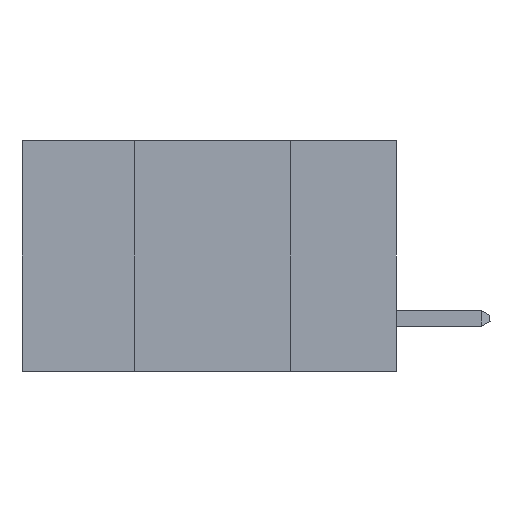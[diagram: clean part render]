
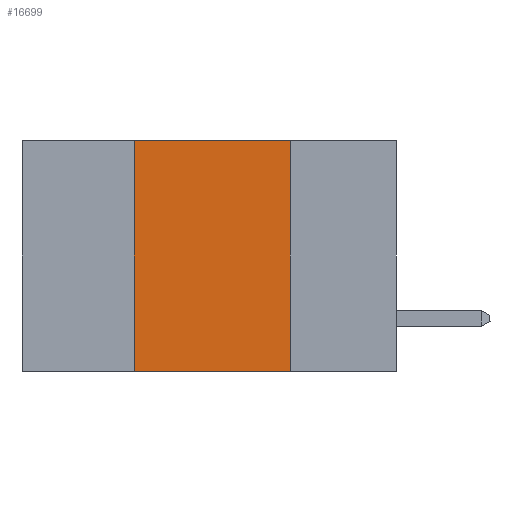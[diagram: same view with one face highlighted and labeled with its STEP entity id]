
A CAD part, left-side view. The second image highlights one B-rep face of the part: STEP entity #16699.
In plain terms, the highlighted planar face has unit normal (-1, 0, 0).
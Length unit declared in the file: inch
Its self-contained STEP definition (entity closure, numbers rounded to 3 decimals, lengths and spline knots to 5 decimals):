
#1188 = VECTOR ( 'NONE', #10572, 39.37008 ) ;
#1836 = ORIENTED_EDGE ( 'NONE', *, *, #16787, .T. ) ;
#1976 = CARTESIAN_POINT ( 'NONE',  ( 0., 0.6, 0. ) ) ;
#2512 = CARTESIAN_POINT ( 'NONE',  ( 0., 0.17, 0. ) ) ;
#2566 = LINE ( 'NONE', #2838, #17258 ) ;
#2645 = DIRECTION ( 'NONE',  ( 1., 0., 0. ) ) ;
#2838 = CARTESIAN_POINT ( 'NONE',  ( 0., 0.6, -0.37 ) ) ;
#2973 = CARTESIAN_POINT ( 'NONE',  ( 0., 0.17, 0. ) ) ;
#5061 = DIRECTION ( 'NONE',  ( 0., 0., 1. ) ) ;
#5926 = EDGE_CURVE ( 'NONE', #7946, #16697, #14800, .T. ) ;
#6313 = LINE ( 'NONE', #2973, #1188 ) ;
#7632 = ORIENTED_EDGE ( 'NONE', *, *, #9331, .F. ) ;
#7685 = DIRECTION ( 'NONE',  ( 0., -1., 0. ) ) ;
#7946 = VERTEX_POINT ( 'NONE', #13555 ) ;
#8011 = ORIENTED_EDGE ( 'NONE', *, *, #18366, .F. ) ;
#8271 = VECTOR ( 'NONE', #7685, 39.37008 ) ;
#9162 = CARTESIAN_POINT ( 'NONE',  ( 0., 0.17, -0.37 ) ) ;
#9331 = EDGE_CURVE ( 'NONE', #13633, #17207, #6313, .T. ) ;
#9452 = FACE_OUTER_BOUND ( 'NONE', #15798, .T. ) ;
#9486 = CARTESIAN_POINT ( 'NONE',  ( 0., 0.42, 0. ) ) ;
#10498 = LINE ( 'NONE', #1976, #8271 ) ;
#10572 = DIRECTION ( 'NONE',  ( 0., 0., -1. ) ) ;
#10965 = VECTOR ( 'NONE', #5061, 39.37008 ) ;
#11191 = CARTESIAN_POINT ( 'NONE',  ( 0., 0.6, 0. ) ) ;
#11433 = DIRECTION ( 'NONE',  ( 0., -1., 0. ) ) ;
#13049 = AXIS2_PLACEMENT_3D ( 'NONE', #11191, #2645, #13829 ) ;
#13555 = CARTESIAN_POINT ( 'NONE',  ( 0., 0.42, -0.37 ) ) ;
#13575 = ORIENTED_EDGE ( 'NONE', *, *, #5926, .F. ) ;
#13633 = VERTEX_POINT ( 'NONE', #2512 ) ;
#13829 = DIRECTION ( 'NONE',  ( 0., 0., -1. ) ) ;
#13892 = CARTESIAN_POINT ( 'NONE',  ( 0., 0.42, 0. ) ) ;
#14800 = LINE ( 'NONE', #9486, #10965 ) ;
#15798 = EDGE_LOOP ( 'NONE', ( #7632, #8011, #13575, #1836 ) ) ;
#16697 = VERTEX_POINT ( 'NONE', #13892 ) ;
#16699 = ADVANCED_FACE ( 'NONE', ( #9452 ), #18104, .F. ) ;
#16787 = EDGE_CURVE ( 'NONE', #7946, #17207, #2566, .T. ) ;
#17207 = VERTEX_POINT ( 'NONE', #9162 ) ;
#17258 = VECTOR ( 'NONE', #11433, 39.37008 ) ;
#18104 = PLANE ( 'NONE',  #13049 ) ;
#18366 = EDGE_CURVE ( 'NONE', #16697, #13633, #10498, .T. ) ;
